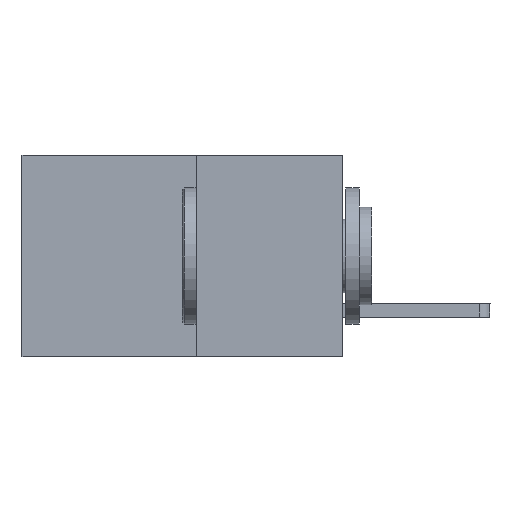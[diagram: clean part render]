
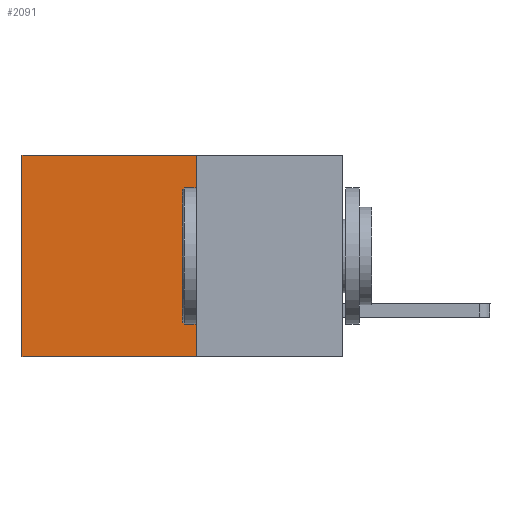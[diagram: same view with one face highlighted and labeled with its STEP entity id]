
A CAD part, left-side view. The second image highlights one B-rep face of the part: STEP entity #2091.
In plain terms, the highlighted planar face has unit normal (-1, 0, 0).
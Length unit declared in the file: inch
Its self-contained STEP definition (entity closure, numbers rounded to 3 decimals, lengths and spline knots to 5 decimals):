
#130 = VERTEX_POINT ( 'NONE', #7005 ) ;
#664 = EDGE_LOOP ( 'NONE', ( #10767, #12220, #12450, #5207 ) ) ;
#945 = CARTESIAN_POINT ( 'NONE',  ( 0.277, 0.27, -0.37 ) ) ;
#2091 = ADVANCED_FACE ( 'NONE', ( #11349 ), #7035, .F. ) ;
#2241 = DIRECTION ( 'NONE',  ( 0., 0., -1. ) ) ;
#2531 = LINE ( 'NONE', #5080, #9939 ) ;
#2564 = LINE ( 'NONE', #4167, #7790 ) ;
#2698 = CARTESIAN_POINT ( 'NONE',  ( 0.277, 0.59, -0.37 ) ) ;
#3759 = EDGE_CURVE ( 'NONE', #6933, #6728, #11587, .T. ) ;
#3862 = DIRECTION ( 'NONE',  ( 0., 0., -1. ) ) ;
#4167 = CARTESIAN_POINT ( 'NONE',  ( 0.277, 0.27, -0.37 ) ) ;
#4178 = DIRECTION ( 'NONE',  ( 0., 1., 0. ) ) ;
#4383 = DIRECTION ( 'NONE',  ( 1., 0., 0. ) ) ;
#4450 = VECTOR ( 'NONE', #3862, 39.37008 ) ;
#4727 = DIRECTION ( 'NONE',  ( 0., 1., 0. ) ) ;
#5060 = EDGE_CURVE ( 'NONE', #10470, #6728, #2564, .T. ) ;
#5080 = CARTESIAN_POINT ( 'NONE',  ( 0.277, 0.27, 0. ) ) ;
#5207 = ORIENTED_EDGE ( 'NONE', *, *, #6970, .T. ) ;
#5894 = CARTESIAN_POINT ( 'NONE',  ( 0.277, 0.59, 0. ) ) ;
#6429 = LINE ( 'NONE', #9560, #4450 ) ;
#6728 = VERTEX_POINT ( 'NONE', #10808 ) ;
#6933 = VERTEX_POINT ( 'NONE', #5894 ) ;
#6970 = EDGE_CURVE ( 'NONE', #130, #6933, #2531, .T. ) ;
#7005 = CARTESIAN_POINT ( 'NONE',  ( 0.277, 0.27, 0. ) ) ;
#7035 = PLANE ( 'NONE',  #12535 ) ;
#7790 = VECTOR ( 'NONE', #4178, 39.37008 ) ;
#9142 = VECTOR ( 'NONE', #2241, 39.37008 ) ;
#9560 = CARTESIAN_POINT ( 'NONE',  ( 0.277, 0.27, -0.37 ) ) ;
#9606 = DIRECTION ( 'NONE',  ( 0., 0., -1. ) ) ;
#9939 = VECTOR ( 'NONE', #4727, 39.37008 ) ;
#10470 = VERTEX_POINT ( 'NONE', #945 ) ;
#10767 = ORIENTED_EDGE ( 'NONE', *, *, #3759, .T. ) ;
#10808 = CARTESIAN_POINT ( 'NONE',  ( 0.277, 0.59, -0.37 ) ) ;
#11286 = CARTESIAN_POINT ( 'NONE',  ( 0.277, 0.27, -0.37 ) ) ;
#11349 = FACE_OUTER_BOUND ( 'NONE', #664, .T. ) ;
#11384 = EDGE_CURVE ( 'NONE', #130, #10470, #6429, .T. ) ;
#11587 = LINE ( 'NONE', #2698, #9142 ) ;
#12220 = ORIENTED_EDGE ( 'NONE', *, *, #5060, .F. ) ;
#12450 = ORIENTED_EDGE ( 'NONE', *, *, #11384, .F. ) ;
#12535 = AXIS2_PLACEMENT_3D ( 'NONE', #11286, #4383, #9606 ) ;
